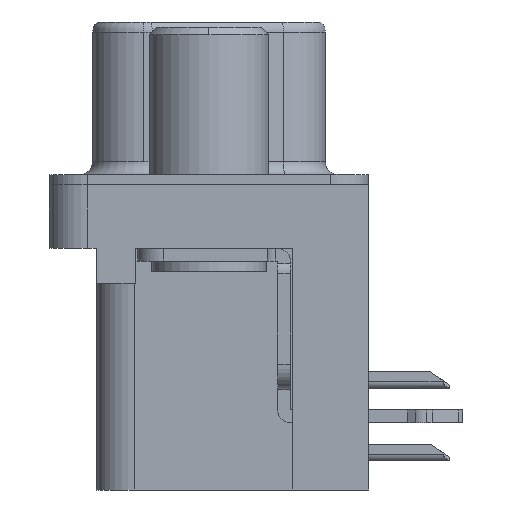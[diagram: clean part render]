
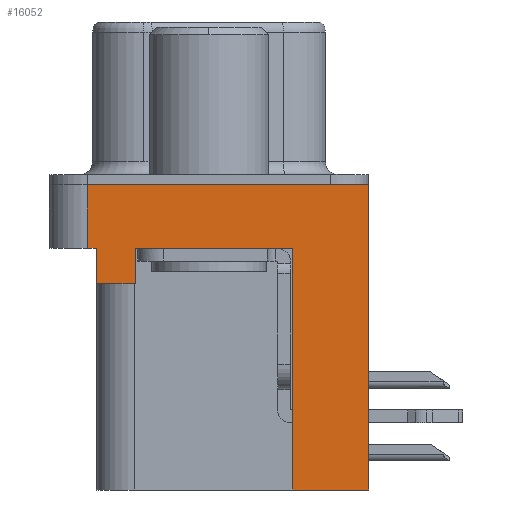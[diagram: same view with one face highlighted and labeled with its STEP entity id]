
A CAD part, left-side view. The second image highlights one B-rep face of the part: STEP entity #16052.
In plain terms, the highlighted planar face has unit normal (-1, 0, 0).
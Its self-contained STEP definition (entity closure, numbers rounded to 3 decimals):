
#499 = DIRECTION ( 'NONE',  ( 0., 0., 1. ) ) ;
#599 = CARTESIAN_POINT ( 'NONE',  ( -2.935, 4.775, 0. ) ) ;
#1085 = EDGE_CURVE ( 'NONE', #4877, #16135, #14843, .T. ) ;
#1725 = EDGE_CURVE ( 'NONE', #19408, #9324, #13150, .T. ) ;
#2313 = EDGE_CURVE ( 'NONE', #19408, #9625, #17639, .T. ) ;
#2403 = VECTOR ( 'NONE', #2455, 1000. ) ;
#2455 = DIRECTION ( 'NONE',  ( 0., 0., 1. ) ) ;
#2510 = CARTESIAN_POINT ( 'NONE',  ( -2.935, -6.275, -2.5 ) ) ;
#2888 = CARTESIAN_POINT ( 'NONE',  ( -2.935, 4.425, -3.9 ) ) ;
#3785 = DIRECTION ( 'NONE',  ( -1., 0., 0. ) ) ;
#3859 = VECTOR ( 'NONE', #4279, 1000. ) ;
#4116 = CARTESIAN_POINT ( 'NONE',  ( -2.935, 4.425, -3.9 ) ) ;
#4147 = DIRECTION ( 'NONE',  ( 0., 0., 1. ) ) ;
#4279 = DIRECTION ( 'NONE',  ( 0., -1., 0. ) ) ;
#4301 = EDGE_LOOP ( 'NONE', ( #6528, #9102, #11471, #10104, #14935, #13579, #8636, #14463, #17318, #18458 ) ) ;
#4846 = VERTEX_POINT ( 'NONE', #10112 ) ;
#4877 = VERTEX_POINT ( 'NONE', #8899 ) ;
#5037 = CARTESIAN_POINT ( 'NONE',  ( -2.935, 4.775, -2.5 ) ) ;
#5386 = LINE ( 'NONE', #4116, #18286 ) ;
#5435 = VECTOR ( 'NONE', #9370, 1000. ) ;
#5658 = DIRECTION ( 'NONE',  ( 0., 0., 1. ) ) ;
#6359 = CARTESIAN_POINT ( 'NONE',  ( -2.935, -3.295, -2.5 ) ) ;
#6528 = ORIENTED_EDGE ( 'NONE', *, *, #18215, .F. ) ;
#6836 = VERTEX_POINT ( 'NONE', #7734 ) ;
#6954 = LINE ( 'NONE', #16275, #3859 ) ;
#7697 = FACE_OUTER_BOUND ( 'NONE', #4301, .T. ) ;
#7734 = CARTESIAN_POINT ( 'NONE',  ( -2.935, -6.275, -12. ) ) ;
#8343 = VERTEX_POINT ( 'NONE', #599 ) ;
#8636 = ORIENTED_EDGE ( 'NONE', *, *, #9169, .T. ) ;
#8670 = DIRECTION ( 'NONE',  ( 0., -1., 0. ) ) ;
#8899 = CARTESIAN_POINT ( 'NONE',  ( -2.935, 4.775, -2.5 ) ) ;
#9102 = ORIENTED_EDGE ( 'NONE', *, *, #10371, .F. ) ;
#9169 = EDGE_CURVE ( 'NONE', #9625, #17704, #11409, .T. ) ;
#9215 = VECTOR ( 'NONE', #4147, 1000. ) ;
#9324 = VERTEX_POINT ( 'NONE', #2888 ) ;
#9367 = CARTESIAN_POINT ( 'NONE',  ( -2.935, -3.295, -12. ) ) ;
#9370 = DIRECTION ( 'NONE',  ( 0., 0., 1. ) ) ;
#9435 = EDGE_CURVE ( 'NONE', #6836, #18955, #10673, .T. ) ;
#9625 = VERTEX_POINT ( 'NONE', #13703 ) ;
#9862 = CARTESIAN_POINT ( 'NONE',  ( -2.935, 4.425, -3.9 ) ) ;
#10104 = ORIENTED_EDGE ( 'NONE', *, *, #13302, .F. ) ;
#10112 = CARTESIAN_POINT ( 'NONE',  ( -2.935, -6.275, 0. ) ) ;
#10371 = EDGE_CURVE ( 'NONE', #4877, #8343, #16107, .T. ) ;
#10532 = VECTOR ( 'NONE', #11359, 1000. ) ;
#10551 = VECTOR ( 'NONE', #8670, 1000. ) ;
#10673 = LINE ( 'NONE', #9367, #19463 ) ;
#11359 = DIRECTION ( 'NONE',  ( 0., 1., 0. ) ) ;
#11409 = LINE ( 'NONE', #11882, #18537 ) ;
#11471 = ORIENTED_EDGE ( 'NONE', *, *, #1085, .T. ) ;
#11604 = EDGE_CURVE ( 'NONE', #18955, #17704, #14034, .T. ) ;
#11882 = CARTESIAN_POINT ( 'NONE',  ( -2.935, -6.275, -2.5 ) ) ;
#12540 = EDGE_CURVE ( 'NONE', #6836, #4846, #14502, .T. ) ;
#12661 = CARTESIAN_POINT ( 'NONE',  ( -2.935, -3.295, -12. ) ) ;
#12900 = CARTESIAN_POINT ( 'NONE',  ( -2.935, -6.275, -2.5 ) ) ;
#12941 = PLANE ( 'NONE',  #18225 ) ;
#13150 = LINE ( 'NONE', #9862, #10532 ) ;
#13302 = EDGE_CURVE ( 'NONE', #9324, #16135, #5386, .T. ) ;
#13579 = ORIENTED_EDGE ( 'NONE', *, *, #2313, .T. ) ;
#13703 = CARTESIAN_POINT ( 'NONE',  ( -2.935, 2.895, -2.5 ) ) ;
#14034 = LINE ( 'NONE', #19508, #5435 ) ;
#14388 = CARTESIAN_POINT ( 'NONE',  ( -2.935, -6.275, -2.5 ) ) ;
#14463 = ORIENTED_EDGE ( 'NONE', *, *, #11604, .F. ) ;
#14502 = LINE ( 'NONE', #2510, #9215 ) ;
#14843 = LINE ( 'NONE', #12900, #10551 ) ;
#14857 = DIRECTION ( 'NONE',  ( 0., 0., 1. ) ) ;
#14935 = ORIENTED_EDGE ( 'NONE', *, *, #1725, .F. ) ;
#15007 = DIRECTION ( 'NONE',  ( 0., -1., 0. ) ) ;
#16052 = ADVANCED_FACE ( 'NONE', ( #7697 ), #12941, .T. ) ;
#16107 = LINE ( 'NONE', #5037, #17402 ) ;
#16135 = VERTEX_POINT ( 'NONE', #16387 ) ;
#16233 = CARTESIAN_POINT ( 'NONE',  ( -2.935, 2.895, -3.9 ) ) ;
#16275 = CARTESIAN_POINT ( 'NONE',  ( -2.935, -6.275, 0. ) ) ;
#16373 = CARTESIAN_POINT ( 'NONE',  ( -2.935, 2.895, -3.9 ) ) ;
#16387 = CARTESIAN_POINT ( 'NONE',  ( -2.935, 4.425, -2.5 ) ) ;
#17306 = DIRECTION ( 'NONE',  ( 0., 1., 0. ) ) ;
#17318 = ORIENTED_EDGE ( 'NONE', *, *, #9435, .F. ) ;
#17402 = VECTOR ( 'NONE', #499, 1000. ) ;
#17639 = LINE ( 'NONE', #16233, #2403 ) ;
#17704 = VERTEX_POINT ( 'NONE', #6359 ) ;
#18215 = EDGE_CURVE ( 'NONE', #8343, #4846, #6954, .T. ) ;
#18225 = AXIS2_PLACEMENT_3D ( 'NONE', #14388, #3785, #14857 ) ;
#18286 = VECTOR ( 'NONE', #5658, 1000. ) ;
#18458 = ORIENTED_EDGE ( 'NONE', *, *, #12540, .T. ) ;
#18537 = VECTOR ( 'NONE', #15007, 1000. ) ;
#18955 = VERTEX_POINT ( 'NONE', #12661 ) ;
#19408 = VERTEX_POINT ( 'NONE', #16373 ) ;
#19463 = VECTOR ( 'NONE', #17306, 1000. ) ;
#19508 = CARTESIAN_POINT ( 'NONE',  ( -2.935, -3.295, -12. ) ) ;
